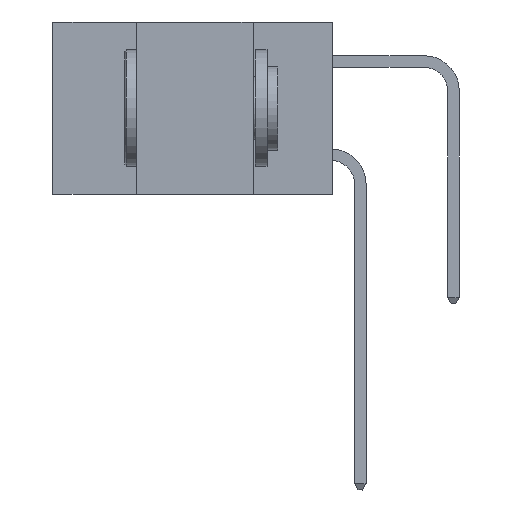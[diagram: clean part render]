
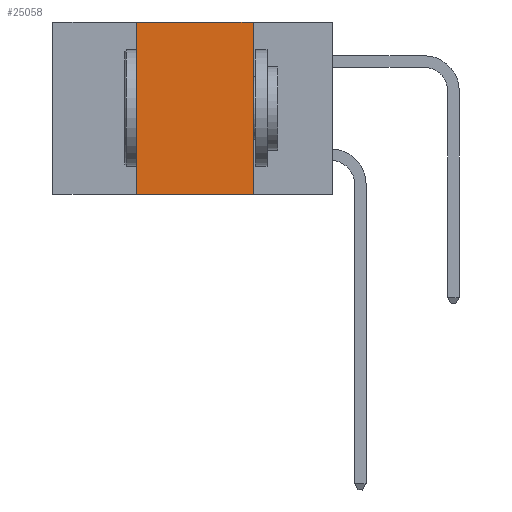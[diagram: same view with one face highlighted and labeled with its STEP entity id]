
A CAD part, left-side view. The second image highlights one B-rep face of the part: STEP entity #25058.
In plain terms, the highlighted planar face has unit normal (-1, 0, 0).
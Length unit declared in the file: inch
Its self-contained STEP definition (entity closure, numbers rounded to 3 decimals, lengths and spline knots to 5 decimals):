
#617 = ORIENTED_EDGE ( 'NONE', *, *, #721, .F. ) ;
#721 = EDGE_CURVE ( 'NONE', #1025, #19333, #16415, .T. ) ;
#937 = LINE ( 'NONE', #11850, #18067 ) ;
#1025 = VERTEX_POINT ( 'NONE', #20514 ) ;
#1410 = DIRECTION ( 'NONE',  ( 0., -1., 0. ) ) ;
#1414 = CARTESIAN_POINT ( 'NONE',  ( 0., 0.6, 0. ) ) ;
#1483 = AXIS2_PLACEMENT_3D ( 'NONE', #1414, #10472, #25891 ) ;
#2247 = EDGE_CURVE ( 'NONE', #6435, #9445, #937, .T. ) ;
#3158 = ORIENTED_EDGE ( 'NONE', *, *, #16426, .F. ) ;
#3442 = VECTOR ( 'NONE', #1410, 39.37008 ) ;
#4166 = LINE ( 'NONE', #12625, #3442 ) ;
#5442 = DIRECTION ( 'NONE',  ( 0., -1., 0. ) ) ;
#6435 = VERTEX_POINT ( 'NONE', #16321 ) ;
#6653 = LINE ( 'NONE', #14325, #24303 ) ;
#8526 = ORIENTED_EDGE ( 'NONE', *, *, #9783, .T. ) ;
#9219 = CARTESIAN_POINT ( 'NONE',  ( 0., 0.17, -0.37 ) ) ;
#9445 = VERTEX_POINT ( 'NONE', #9219 ) ;
#9783 = EDGE_CURVE ( 'NONE', #1025, #9445, #4166, .T. ) ;
#10472 = DIRECTION ( 'NONE',  ( 1., 0., 0. ) ) ;
#11850 = CARTESIAN_POINT ( 'NONE',  ( 0., 0.17, 0. ) ) ;
#12625 = CARTESIAN_POINT ( 'NONE',  ( 0., 0.6, -0.37 ) ) ;
#13831 = CARTESIAN_POINT ( 'NONE',  ( 0., 0.42, 0. ) ) ;
#14325 = CARTESIAN_POINT ( 'NONE',  ( 0., 0.6, 0. ) ) ;
#16321 = CARTESIAN_POINT ( 'NONE',  ( 0., 0.17, 0. ) ) ;
#16415 = LINE ( 'NONE', #25252, #22250 ) ;
#16426 = EDGE_CURVE ( 'NONE', #19333, #6435, #6653, .T. ) ;
#17645 = EDGE_LOOP ( 'NONE', ( #27372, #3158, #617, #8526 ) ) ;
#18067 = VECTOR ( 'NONE', #23665, 39.37008 ) ;
#19333 = VERTEX_POINT ( 'NONE', #13831 ) ;
#20514 = CARTESIAN_POINT ( 'NONE',  ( 0., 0.42, -0.37 ) ) ;
#21062 = FACE_OUTER_BOUND ( 'NONE', #17645, .T. ) ;
#22250 = VECTOR ( 'NONE', #23937, 39.37008 ) ;
#23656 = PLANE ( 'NONE',  #1483 ) ;
#23665 = DIRECTION ( 'NONE',  ( 0., 0., -1. ) ) ;
#23937 = DIRECTION ( 'NONE',  ( 0., 0., 1. ) ) ;
#24303 = VECTOR ( 'NONE', #5442, 39.37008 ) ;
#25058 = ADVANCED_FACE ( 'NONE', ( #21062 ), #23656, .F. ) ;
#25252 = CARTESIAN_POINT ( 'NONE',  ( 0., 0.42, 0. ) ) ;
#25891 = DIRECTION ( 'NONE',  ( 0., 0., -1. ) ) ;
#27372 = ORIENTED_EDGE ( 'NONE', *, *, #2247, .F. ) ;
